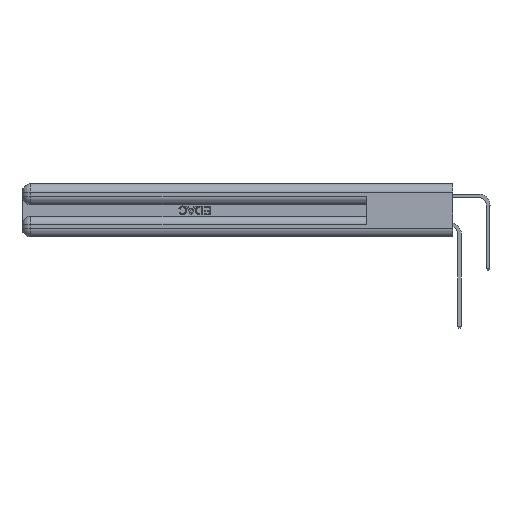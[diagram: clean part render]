
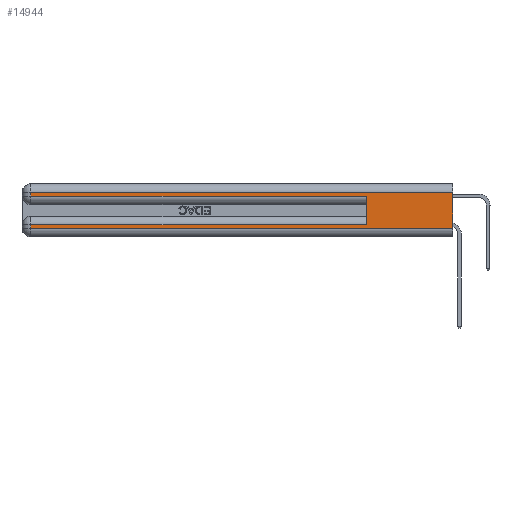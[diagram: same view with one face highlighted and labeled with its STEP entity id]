
A CAD part, left-side view. The second image highlights one B-rep face of the part: STEP entity #14944.
In plain terms, the highlighted planar face has unit normal (-1, 0, 0).
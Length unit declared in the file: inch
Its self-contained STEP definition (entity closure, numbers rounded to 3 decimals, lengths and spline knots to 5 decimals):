
#405 = EDGE_CURVE ( 'NONE', #17162, #15926, #23002, .T. ) ;
#1867 = VERTEX_POINT ( 'NONE', #22721 ) ;
#2007 = ORIENTED_EDGE ( 'NONE', *, *, #16059, .T. ) ;
#3161 = DIRECTION ( 'NONE',  ( 0., -1., 0. ) ) ;
#4548 = VECTOR ( 'NONE', #43932, 39.37008 ) ;
#4750 = ORIENTED_EDGE ( 'NONE', *, *, #30079, .T. ) ;
#4908 = LINE ( 'NONE', #24791, #35821 ) ;
#6599 = DIRECTION ( 'NONE',  ( 0., 0., 1. ) ) ;
#6789 = CARTESIAN_POINT ( 'NONE',  ( 0., 2.94, 0.37 ) ) ;
#7091 = PLANE ( 'NONE',  #28202 ) ;
#7882 = CARTESIAN_POINT ( 'NONE',  ( 0., 0., 0.06 ) ) ;
#8482 = ORIENTED_EDGE ( 'NONE', *, *, #19305, .T. ) ;
#9056 = ORIENTED_EDGE ( 'NONE', *, *, #18038, .F. ) ;
#9262 = CARTESIAN_POINT ( 'NONE',  ( 0., 0., 0.285 ) ) ;
#9613 = FACE_OUTER_BOUND ( 'NONE', #27447, .T. ) ;
#9741 = VECTOR ( 'NONE', #3161, 39.37008 ) ;
#10660 = VECTOR ( 'NONE', #42565, 39.37008 ) ;
#10727 = EDGE_CURVE ( 'NONE', #27428, #29773, #42571, .T. ) ;
#10757 = CARTESIAN_POINT ( 'NONE',  ( 0., 2.94, 0.31 ) ) ;
#11319 = ORIENTED_EDGE ( 'NONE', *, *, #20384, .T. ) ;
#12500 = EDGE_CURVE ( 'NONE', #37852, #21671, #4908, .T. ) ;
#12812 = DIRECTION ( 'NONE',  ( 0., 1., 0. ) ) ;
#13315 = CARTESIAN_POINT ( 'NONE',  ( 0., 2.94, 0.285 ) ) ;
#14507 = CARTESIAN_POINT ( 'NONE',  ( 0., 0., 0.37 ) ) ;
#14944 = ADVANCED_FACE ( 'NONE', ( #9613 ), #7091, .F. ) ;
#15775 = VECTOR ( 'NONE', #12812, 39.37008 ) ;
#15926 = VERTEX_POINT ( 'NONE', #7882 ) ;
#16059 = EDGE_CURVE ( 'NONE', #37852, #30396, #32714, .T. ) ;
#16650 = VECTOR ( 'NONE', #32241, 39.37008 ) ;
#16688 = CARTESIAN_POINT ( 'NONE',  ( 0., 0., 0.31 ) ) ;
#17162 = VERTEX_POINT ( 'NONE', #20773 ) ;
#18038 = EDGE_CURVE ( 'NONE', #1867, #15926, #26388, .T. ) ;
#19249 = CARTESIAN_POINT ( 'NONE',  ( 0., 0., 0.085 ) ) ;
#19305 = EDGE_CURVE ( 'NONE', #1867, #27428, #25105, .T. ) ;
#20384 = EDGE_CURVE ( 'NONE', #29773, #21671, #38308, .T. ) ;
#20543 = CARTESIAN_POINT ( 'NONE',  ( 0., 0.6, 0.085 ) ) ;
#20773 = CARTESIAN_POINT ( 'NONE',  ( 0., 2.94, 0.06 ) ) ;
#21671 = VERTEX_POINT ( 'NONE', #28172 ) ;
#21715 = ORIENTED_EDGE ( 'NONE', *, *, #405, .T. ) ;
#22721 = CARTESIAN_POINT ( 'NONE',  ( 0., 0., 0.31 ) ) ;
#23002 = LINE ( 'NONE', #36555, #9741 ) ;
#24582 = ORIENTED_EDGE ( 'NONE', *, *, #12500, .F. ) ;
#24791 = CARTESIAN_POINT ( 'NONE',  ( 0., 0.6, 0.145 ) ) ;
#25105 = LINE ( 'NONE', #16688, #15775 ) ;
#26388 = LINE ( 'NONE', #14507, #34668 ) ;
#26521 = CARTESIAN_POINT ( 'NONE',  ( 0., 2.94, 0.085 ) ) ;
#27428 = VERTEX_POINT ( 'NONE', #10757 ) ;
#27447 = EDGE_LOOP ( 'NONE', ( #9056, #8482, #30429, #11319, #24582, #2007, #4750, #21715 ) ) ;
#28172 = CARTESIAN_POINT ( 'NONE',  ( 0., 0.6, 0.285 ) ) ;
#28202 = AXIS2_PLACEMENT_3D ( 'NONE', #34764, #38771, #42147 ) ;
#29773 = VERTEX_POINT ( 'NONE', #13315 ) ;
#30079 = EDGE_CURVE ( 'NONE', #30396, #17162, #43843, .T. ) ;
#30396 = VERTEX_POINT ( 'NONE', #26521 ) ;
#30429 = ORIENTED_EDGE ( 'NONE', *, *, #10727, .T. ) ;
#32241 = DIRECTION ( 'NONE',  ( 0., 0., -1. ) ) ;
#32361 = CARTESIAN_POINT ( 'NONE',  ( 0., 2.94, 0.37 ) ) ;
#32714 = LINE ( 'NONE', #19249, #4548 ) ;
#34668 = VECTOR ( 'NONE', #39216, 39.37008 ) ;
#34764 = CARTESIAN_POINT ( 'NONE',  ( 0., 0., 0.37 ) ) ;
#35821 = VECTOR ( 'NONE', #6599, 39.37008 ) ;
#36080 = VECTOR ( 'NONE', #37393, 39.37008 ) ;
#36555 = CARTESIAN_POINT ( 'NONE',  ( 0., 0., 0.06 ) ) ;
#37393 = DIRECTION ( 'NONE',  ( 0., -1., 0. ) ) ;
#37852 = VERTEX_POINT ( 'NONE', #20543 ) ;
#38308 = LINE ( 'NONE', #9262, #36080 ) ;
#38771 = DIRECTION ( 'NONE',  ( 1., 0., 0. ) ) ;
#39216 = DIRECTION ( 'NONE',  ( 0., 0., -1. ) ) ;
#42147 = DIRECTION ( 'NONE',  ( 0., 0., -1. ) ) ;
#42565 = DIRECTION ( 'NONE',  ( 0., 0., -1. ) ) ;
#42571 = LINE ( 'NONE', #6789, #16650 ) ;
#43843 = LINE ( 'NONE', #32361, #10660 ) ;
#43932 = DIRECTION ( 'NONE',  ( 0., 1., 0. ) ) ;
